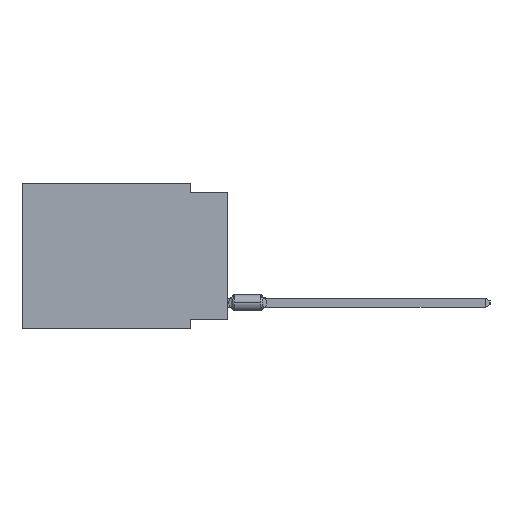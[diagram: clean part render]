
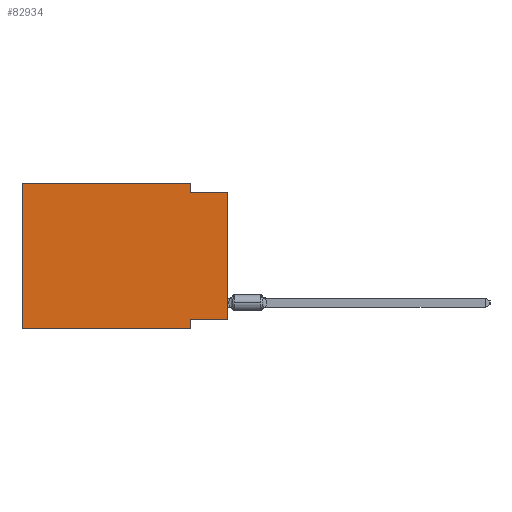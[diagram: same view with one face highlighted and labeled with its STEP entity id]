
A CAD part, left-side view. The second image highlights one B-rep face of the part: STEP entity #82934.
In plain terms, the highlighted planar face has unit normal (-1, 0, 0).
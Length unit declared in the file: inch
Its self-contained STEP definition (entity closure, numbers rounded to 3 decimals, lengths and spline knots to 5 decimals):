
#1455 = ORIENTED_EDGE ( 'NONE', *, *, #3651, .F. ) ;
#2125 = VERTEX_POINT ( 'NONE', #41054 ) ;
#3345 = LINE ( 'NONE', #3752, #4124 ) ;
#3651 = EDGE_CURVE ( 'NONE', #2125, #82099, #20309, .T. ) ;
#3752 = CARTESIAN_POINT ( 'NONE',  ( 0., 0., -0.025 ) ) ;
#4124 = VECTOR ( 'NONE', #29275, 39.37008 ) ;
#4453 = ORIENTED_EDGE ( 'NONE', *, *, #53402, .F. ) ;
#5382 = VERTEX_POINT ( 'NONE', #7468 ) ;
#7468 = CARTESIAN_POINT ( 'NONE',  ( 0., 0.1, 0. ) ) ;
#8672 = VECTOR ( 'NONE', #43210, 39.37008 ) ;
#11040 = ORIENTED_EDGE ( 'NONE', *, *, #61220, .F. ) ;
#18479 = VERTEX_POINT ( 'NONE', #63963 ) ;
#20309 = LINE ( 'NONE', #52603, #44510 ) ;
#20336 = LINE ( 'NONE', #20754, #68370 ) ;
#20754 = CARTESIAN_POINT ( 'NONE',  ( 0., 0.1, 0. ) ) ;
#24798 = PLANE ( 'NONE',  #68167 ) ;
#25641 = CARTESIAN_POINT ( 'NONE',  ( 0., 0.55, 0. ) ) ;
#27195 = VECTOR ( 'NONE', #45556, 39.37008 ) ;
#29275 = DIRECTION ( 'NONE',  ( 0., -1., 0. ) ) ;
#31290 = DIRECTION ( 'NONE',  ( 0., -1., 0. ) ) ;
#32145 = EDGE_CURVE ( 'NONE', #49426, #64489, #3345, .T. ) ;
#34049 = LINE ( 'NONE', #77818, #27195 ) ;
#35171 = LINE ( 'NONE', #43644, #51943 ) ;
#36524 = CARTESIAN_POINT ( 'NONE',  ( 0., 0.55, 0. ) ) ;
#36650 = ORIENTED_EDGE ( 'NONE', *, *, #77853, .T. ) ;
#40921 = CARTESIAN_POINT ( 'NONE',  ( 0., 0.55, 0. ) ) ;
#41054 = CARTESIAN_POINT ( 'NONE',  ( 0., 0., -0.365 ) ) ;
#43210 = DIRECTION ( 'NONE',  ( 0., 0., 1. ) ) ;
#43644 = CARTESIAN_POINT ( 'NONE',  ( 0., 0.55, -0.39 ) ) ;
#44510 = VECTOR ( 'NONE', #45821, 39.37008 ) ;
#44544 = CARTESIAN_POINT ( 'NONE',  ( 0., 0.55, -0.39 ) ) ;
#44771 = FACE_OUTER_BOUND ( 'NONE', #62505, .T. ) ;
#45556 = DIRECTION ( 'NONE',  ( 0., 0., -1. ) ) ;
#45821 = DIRECTION ( 'NONE',  ( 0., 1., 0. ) ) ;
#46398 = VECTOR ( 'NONE', #54587, 39.37008 ) ;
#46545 = ORIENTED_EDGE ( 'NONE', *, *, #72092, .F. ) ;
#49426 = VERTEX_POINT ( 'NONE', #57069 ) ;
#49989 = LINE ( 'NONE', #75875, #8672 ) ;
#50722 = DIRECTION ( 'NONE',  ( 0., 0., -1. ) ) ;
#51943 = VECTOR ( 'NONE', #31290, 39.37008 ) ;
#52167 = VECTOR ( 'NONE', #53226, 39.37008 ) ;
#52603 = CARTESIAN_POINT ( 'NONE',  ( 0., 0., -0.365 ) ) ;
#53226 = DIRECTION ( 'NONE',  ( 0., 0., 1. ) ) ;
#53402 = EDGE_CURVE ( 'NONE', #80099, #74047, #74008, .T. ) ;
#54587 = DIRECTION ( 'NONE',  ( 0., -1., 0. ) ) ;
#55221 = ORIENTED_EDGE ( 'NONE', *, *, #83496, .T. ) ;
#57069 = CARTESIAN_POINT ( 'NONE',  ( 0., 0.1, -0.025 ) ) ;
#61220 = EDGE_CURVE ( 'NONE', #74047, #5382, #66494, .T. ) ;
#62505 = EDGE_LOOP ( 'NONE', ( #36650, #65748, #73452, #11040, #4453, #55221, #46545, #1455 ) ) ;
#63963 = CARTESIAN_POINT ( 'NONE',  ( 0., 0.1, -0.39 ) ) ;
#64489 = VERTEX_POINT ( 'NONE', #67177 ) ;
#65748 = ORIENTED_EDGE ( 'NONE', *, *, #32145, .F. ) ;
#66137 = EDGE_CURVE ( 'NONE', #5382, #49426, #20336, .T. ) ;
#66494 = LINE ( 'NONE', #79227, #46398 ) ;
#67177 = CARTESIAN_POINT ( 'NONE',  ( 0., 0., -0.025 ) ) ;
#68167 = AXIS2_PLACEMENT_3D ( 'NONE', #25641, #77892, #50722 ) ;
#68370 = VECTOR ( 'NONE', #80180, 39.37008 ) ;
#72092 = EDGE_CURVE ( 'NONE', #82099, #18479, #34049, .T. ) ;
#72141 = CARTESIAN_POINT ( 'NONE',  ( 0., 0.1, -0.365 ) ) ;
#73452 = ORIENTED_EDGE ( 'NONE', *, *, #66137, .F. ) ;
#74008 = LINE ( 'NONE', #40921, #52167 ) ;
#74047 = VERTEX_POINT ( 'NONE', #36524 ) ;
#75875 = CARTESIAN_POINT ( 'NONE',  ( 0., 0., 0. ) ) ;
#77818 = CARTESIAN_POINT ( 'NONE',  ( 0., 0.1, -0.39 ) ) ;
#77853 = EDGE_CURVE ( 'NONE', #2125, #64489, #49989, .T. ) ;
#77892 = DIRECTION ( 'NONE',  ( 1., 0., 0. ) ) ;
#79227 = CARTESIAN_POINT ( 'NONE',  ( 0., 0.55, 0. ) ) ;
#80099 = VERTEX_POINT ( 'NONE', #44544 ) ;
#80180 = DIRECTION ( 'NONE',  ( 0., 0., -1. ) ) ;
#82099 = VERTEX_POINT ( 'NONE', #72141 ) ;
#82934 = ADVANCED_FACE ( 'NONE', ( #44771 ), #24798, .F. ) ;
#83496 = EDGE_CURVE ( 'NONE', #80099, #18479, #35171, .T. ) ;
